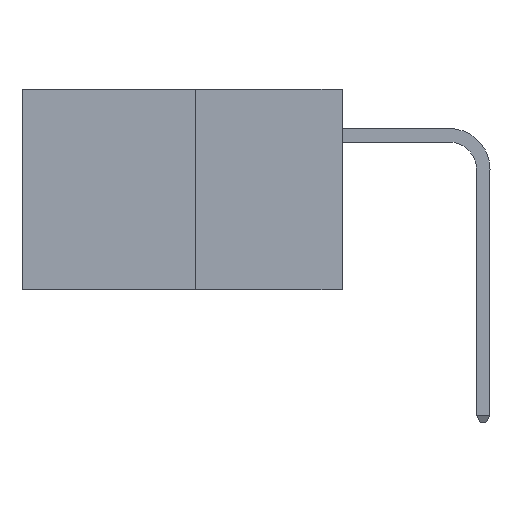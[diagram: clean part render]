
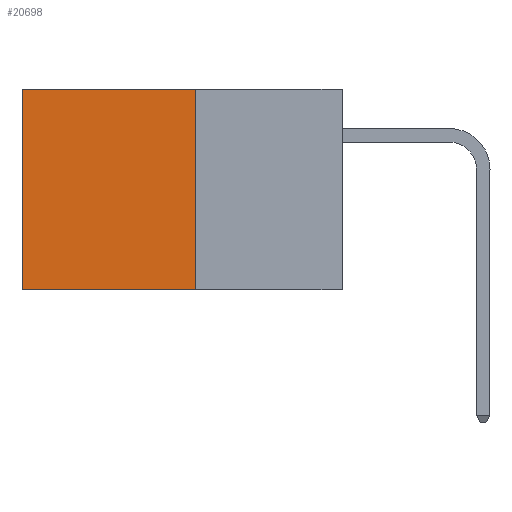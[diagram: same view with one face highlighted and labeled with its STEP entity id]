
A CAD part, left-side view. The second image highlights one B-rep face of the part: STEP entity #20698.
In plain terms, the highlighted planar face has unit normal (-1, 0, 0).
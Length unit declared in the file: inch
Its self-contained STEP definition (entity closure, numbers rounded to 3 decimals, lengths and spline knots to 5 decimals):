
#208 = ORIENTED_EDGE ( 'NONE', *, *, #8281, .T. ) ;
#546 = VECTOR ( 'NONE', #22617, 39.37008 ) ;
#629 = CARTESIAN_POINT ( 'NONE',  ( 0.277, 0.59, -0.37 ) ) ;
#4058 = PLANE ( 'NONE',  #14117 ) ;
#4130 = VERTEX_POINT ( 'NONE', #19096 ) ;
#4267 = EDGE_CURVE ( 'NONE', #4130, #10659, #9447, .T. ) ;
#4759 = DIRECTION ( 'NONE',  ( 0., 1., 0. ) ) ;
#6587 = CARTESIAN_POINT ( 'NONE',  ( 0.277, 0.59, -0.37 ) ) ;
#6614 = LINE ( 'NONE', #16984, #15403 ) ;
#6900 = ORIENTED_EDGE ( 'NONE', *, *, #4267, .F. ) ;
#6913 = LINE ( 'NONE', #21598, #15710 ) ;
#8281 = EDGE_CURVE ( 'NONE', #18848, #17898, #14682, .T. ) ;
#9279 = ORIENTED_EDGE ( 'NONE', *, *, #20038, .F. ) ;
#9447 = LINE ( 'NONE', #9695, #18148 ) ;
#9451 = DIRECTION ( 'NONE',  ( 1., 0., 0. ) ) ;
#9695 = CARTESIAN_POINT ( 'NONE',  ( 0.277, 0.27, -0.37 ) ) ;
#9745 = EDGE_LOOP ( 'NONE', ( #208, #9279, #6900, #15803 ) ) ;
#10659 = VERTEX_POINT ( 'NONE', #19189 ) ;
#10788 = FACE_OUTER_BOUND ( 'NONE', #9745, .T. ) ;
#14117 = AXIS2_PLACEMENT_3D ( 'NONE', #19827, #9451, #21567 ) ;
#14682 = LINE ( 'NONE', #629, #546 ) ;
#15403 = VECTOR ( 'NONE', #4759, 39.37008 ) ;
#15710 = VECTOR ( 'NONE', #21673, 39.37008 ) ;
#15803 = ORIENTED_EDGE ( 'NONE', *, *, #20251, .T. ) ;
#15839 = CARTESIAN_POINT ( 'NONE',  ( 0.277, 0.59, 0. ) ) ;
#16984 = CARTESIAN_POINT ( 'NONE',  ( 0.277, 0.27, 0. ) ) ;
#17475 = DIRECTION ( 'NONE',  ( 0., 0., -1. ) ) ;
#17898 = VERTEX_POINT ( 'NONE', #6587 ) ;
#18148 = VECTOR ( 'NONE', #17475, 39.37008 ) ;
#18848 = VERTEX_POINT ( 'NONE', #15839 ) ;
#19096 = CARTESIAN_POINT ( 'NONE',  ( 0.277, 0.27, 0. ) ) ;
#19189 = CARTESIAN_POINT ( 'NONE',  ( 0.277, 0.27, -0.37 ) ) ;
#19827 = CARTESIAN_POINT ( 'NONE',  ( 0.277, 0.27, -0.37 ) ) ;
#20038 = EDGE_CURVE ( 'NONE', #10659, #17898, #6913, .T. ) ;
#20251 = EDGE_CURVE ( 'NONE', #4130, #18848, #6614, .T. ) ;
#20698 = ADVANCED_FACE ( 'NONE', ( #10788 ), #4058, .F. ) ;
#21567 = DIRECTION ( 'NONE',  ( 0., 0., -1. ) ) ;
#21598 = CARTESIAN_POINT ( 'NONE',  ( 0.277, 0.27, -0.37 ) ) ;
#21673 = DIRECTION ( 'NONE',  ( 0., 1., 0. ) ) ;
#22617 = DIRECTION ( 'NONE',  ( 0., 0., -1. ) ) ;
